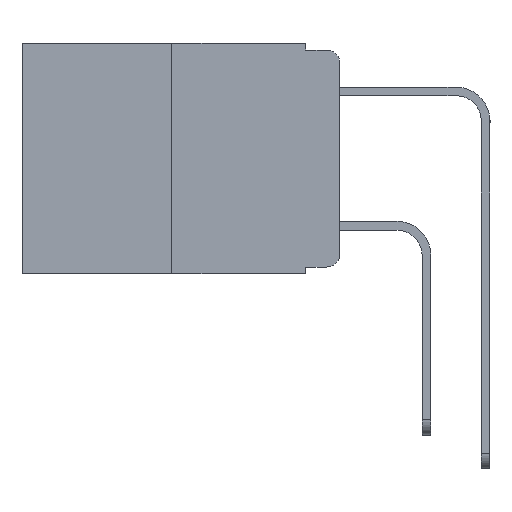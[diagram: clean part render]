
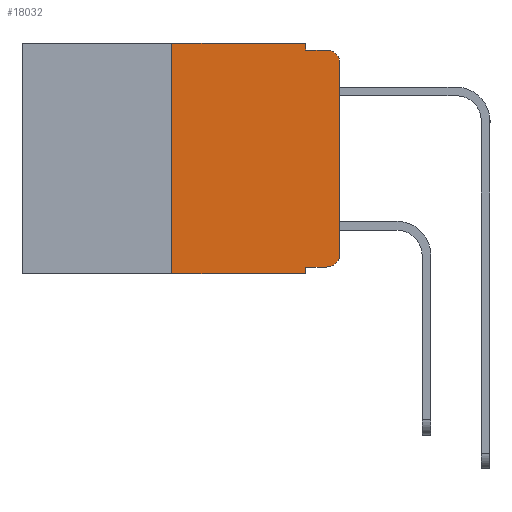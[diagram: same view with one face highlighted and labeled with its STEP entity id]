
A CAD part, left-side view. The second image highlights one B-rep face of the part: STEP entity #18032.
In plain terms, the highlighted planar face has unit normal (-1, 0, 0).
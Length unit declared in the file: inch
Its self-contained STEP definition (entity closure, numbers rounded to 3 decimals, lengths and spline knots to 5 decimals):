
#120 = CARTESIAN_POINT ( 'NONE',  ( 0., 0.473, 0. ) ) ;
#236 = VERTEX_POINT ( 'NONE', #3861 ) ;
#664 = CARTESIAN_POINT ( 'NONE',  ( 0., 0.473, 0. ) ) ;
#681 = CARTESIAN_POINT ( 'NONE',  ( 0., 0.051, -0.343 ) ) ;
#694 = ORIENTED_EDGE ( 'NONE', *, *, #8810, .T. ) ;
#735 = DIRECTION ( 'NONE',  ( 1., 0., 0. ) ) ;
#935 = DIRECTION ( 'NONE',  ( 0., -1., 0. ) ) ;
#939 = EDGE_CURVE ( 'NONE', #2779, #10673, #2971, .T. ) ;
#1672 = CIRCLE ( 'NONE', #2771, 0.02 ) ;
#2036 = VECTOR ( 'NONE', #17227, 39.37008 ) ;
#2352 = CARTESIAN_POINT ( 'NONE',  ( 0., 0.051, -0.01 ) ) ;
#2603 = ORIENTED_EDGE ( 'NONE', *, *, #18113, .T. ) ;
#2771 = AXIS2_PLACEMENT_3D ( 'NONE', #12596, #4210, #13962 ) ;
#2779 = VERTEX_POINT ( 'NONE', #9010 ) ;
#2971 = LINE ( 'NONE', #17286, #2036 ) ;
#3085 = ORIENTED_EDGE ( 'NONE', *, *, #17256, .T. ) ;
#3432 = CARTESIAN_POINT ( 'NONE',  ( 0., 0.051, 0. ) ) ;
#3637 = LINE ( 'NONE', #5680, #14376 ) ;
#3861 = CARTESIAN_POINT ( 'NONE',  ( 0., 0.051, 0. ) ) ;
#3987 = EDGE_CURVE ( 'NONE', #4558, #8211, #6508, .T. ) ;
#4210 = DIRECTION ( 'NONE',  ( -1., 0., 0. ) ) ;
#4347 = CIRCLE ( 'NONE', #17378, 0.02 ) ;
#4552 = VERTEX_POINT ( 'NONE', #14281 ) ;
#4558 = VERTEX_POINT ( 'NONE', #12411 ) ;
#4619 = VECTOR ( 'NONE', #14653, 39.37008 ) ;
#4918 = EDGE_CURVE ( 'NONE', #8211, #236, #10573, .T. ) ;
#4985 = EDGE_CURVE ( 'NONE', #236, #9773, #5079, .T. ) ;
#5079 = LINE ( 'NONE', #3432, #4619 ) ;
#5190 = ORIENTED_EDGE ( 'NONE', *, *, #4985, .F. ) ;
#5680 = CARTESIAN_POINT ( 'NONE',  ( 0., 0.051, -0.01 ) ) ;
#5998 = EDGE_CURVE ( 'NONE', #9773, #13603, #3637, .T. ) ;
#6001 = DIRECTION ( 'NONE',  ( 0., -1., 0. ) ) ;
#6086 = CARTESIAN_POINT ( 'NONE',  ( 0., 0.02, -0.333 ) ) ;
#6259 = DIRECTION ( 'NONE',  ( 0., 0., 1. ) ) ;
#6508 = LINE ( 'NONE', #14523, #14225 ) ;
#6863 = LINE ( 'NONE', #12874, #9656 ) ;
#7521 = CARTESIAN_POINT ( 'NONE',  ( 0., 0.02, -0.313 ) ) ;
#7883 = EDGE_CURVE ( 'NONE', #4552, #13603, #1672, .T. ) ;
#8147 = LINE ( 'NONE', #17675, #18011 ) ;
#8211 = VERTEX_POINT ( 'NONE', #9188 ) ;
#8526 = DIRECTION ( 'NONE',  ( 0., -1., 0. ) ) ;
#8533 = ORIENTED_EDGE ( 'NONE', *, *, #7883, .T. ) ;
#8810 = EDGE_CURVE ( 'NONE', #10056, #4552, #10017, .T. ) ;
#8910 = DIRECTION ( 'NONE',  ( 0., 0., -1. ) ) ;
#8941 = EDGE_LOOP ( 'NONE', ( #694, #8533, #12152, #5190, #8961, #13028, #16560, #16975, #2603, #3085 ) ) ;
#8961 = ORIENTED_EDGE ( 'NONE', *, *, #4918, .F. ) ;
#9010 = CARTESIAN_POINT ( 'NONE',  ( 0., 0.051, -0.333 ) ) ;
#9188 = CARTESIAN_POINT ( 'NONE',  ( 0., 0.25, 0. ) ) ;
#9412 = CARTESIAN_POINT ( 'NONE',  ( 0., 0.02, -0.01 ) ) ;
#9470 = PLANE ( 'NONE',  #13984 ) ;
#9656 = VECTOR ( 'NONE', #6001, 39.37008 ) ;
#9773 = VERTEX_POINT ( 'NONE', #2352 ) ;
#10017 = LINE ( 'NONE', #11728, #13218 ) ;
#10050 = VERTEX_POINT ( 'NONE', #6086 ) ;
#10056 = VERTEX_POINT ( 'NONE', #10263 ) ;
#10263 = CARTESIAN_POINT ( 'NONE',  ( 0., 0., -0.313 ) ) ;
#10573 = LINE ( 'NONE', #120, #11427 ) ;
#10673 = VERTEX_POINT ( 'NONE', #681 ) ;
#10840 = DIRECTION ( 'NONE',  ( 0., 0., -1. ) ) ;
#11427 = VECTOR ( 'NONE', #11712, 39.37008 ) ;
#11712 = DIRECTION ( 'NONE',  ( 0., -1., 0. ) ) ;
#11728 = CARTESIAN_POINT ( 'NONE',  ( 0., 0., 0. ) ) ;
#12152 = ORIENTED_EDGE ( 'NONE', *, *, #5998, .F. ) ;
#12411 = CARTESIAN_POINT ( 'NONE',  ( 0., 0.25, -0.343 ) ) ;
#12596 = CARTESIAN_POINT ( 'NONE',  ( 0., 0.02, -0.03 ) ) ;
#12639 = FACE_OUTER_BOUND ( 'NONE', #8941, .T. ) ;
#12874 = CARTESIAN_POINT ( 'NONE',  ( 0., 0.473, -0.343 ) ) ;
#13028 = ORIENTED_EDGE ( 'NONE', *, *, #3987, .F. ) ;
#13218 = VECTOR ( 'NONE', #6259, 39.37008 ) ;
#13603 = VERTEX_POINT ( 'NONE', #9412 ) ;
#13835 = DIRECTION ( 'NONE',  ( 0., 0., 1. ) ) ;
#13936 = EDGE_CURVE ( 'NONE', #4558, #10673, #6863, .T. ) ;
#13962 = DIRECTION ( 'NONE',  ( 0., 0., -1. ) ) ;
#13984 = AXIS2_PLACEMENT_3D ( 'NONE', #664, #735, #10840 ) ;
#14225 = VECTOR ( 'NONE', #13835, 39.37008 ) ;
#14281 = CARTESIAN_POINT ( 'NONE',  ( 0., 0., -0.03 ) ) ;
#14376 = VECTOR ( 'NONE', #8526, 39.37008 ) ;
#14523 = CARTESIAN_POINT ( 'NONE',  ( 0., 0.25, 0. ) ) ;
#14653 = DIRECTION ( 'NONE',  ( 0., 0., -1. ) ) ;
#16560 = ORIENTED_EDGE ( 'NONE', *, *, #13936, .T. ) ;
#16975 = ORIENTED_EDGE ( 'NONE', *, *, #939, .F. ) ;
#16977 = DIRECTION ( 'NONE',  ( -1., 0., 0. ) ) ;
#17227 = DIRECTION ( 'NONE',  ( 0., 0., -1. ) ) ;
#17256 = EDGE_CURVE ( 'NONE', #10050, #10056, #4347, .T. ) ;
#17286 = CARTESIAN_POINT ( 'NONE',  ( 0., 0.051, 0. ) ) ;
#17378 = AXIS2_PLACEMENT_3D ( 'NONE', #7521, #16977, #8910 ) ;
#17675 = CARTESIAN_POINT ( 'NONE',  ( 0., 0.051, -0.333 ) ) ;
#18011 = VECTOR ( 'NONE', #935, 39.37008 ) ;
#18032 = ADVANCED_FACE ( 'NONE', ( #12639 ), #9470, .F. ) ;
#18113 = EDGE_CURVE ( 'NONE', #2779, #10050, #8147, .T. ) ;
